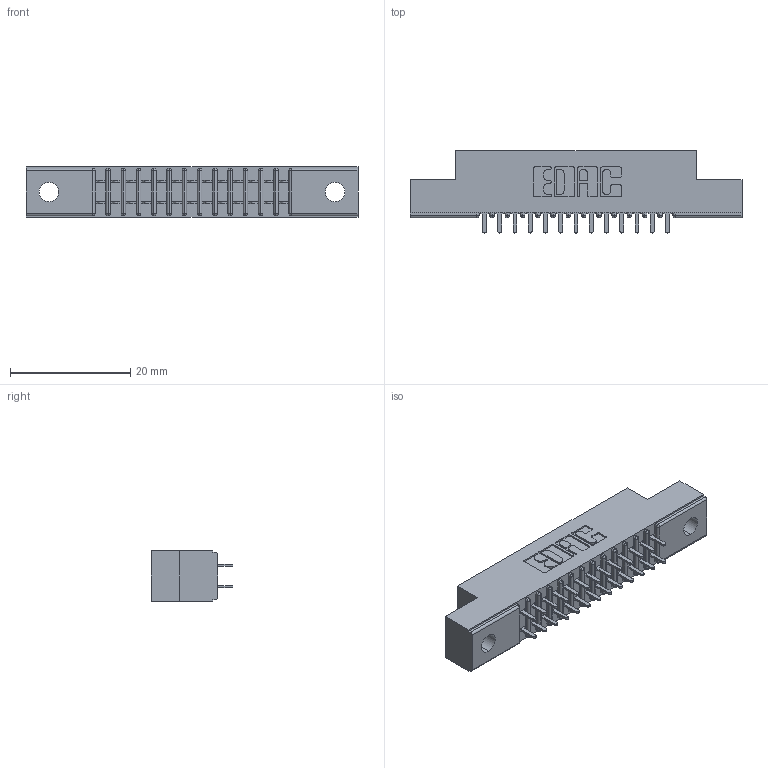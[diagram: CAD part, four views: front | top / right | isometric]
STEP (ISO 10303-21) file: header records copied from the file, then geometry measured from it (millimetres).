
FILE_DESCRIPTION (( 'STEP AP203' ), '1' );
FILE_NAME ('391-026-524-202.STEP', '2018-08-08T20:27:36', ( '' ), ( '' ), 'SwSTEP 2.0', 'SolidWorks 2016', '' );
FILE_SCHEMA (( 'CONFIG_CONTROL_DESIGN' ));
Length unit declared in the file: inch
Products named in the file (3): 341 Part_.128 (3.25) Dia Mounting Holes; 341-292-001_341-292-124; 391-026-524-202
Assembly tree (27 placements, depth 2):
  391-026-524-202
    341 Part_.128 (3.25) Dia Mounting Holes
    341-292-001_341-292-124  x26
Bounding box: 55.24 x 13.64 x 8.38 mm (x, y, z)
Volume: 3127.1 mm3; surface area: 5671.1 mm2
Topology: 27 solids, 27 shells, 1832 faces, 5295 edges, 3430 vertices
Faces by surface type: plane 1108, cylinder 672, sphere 28, torus 24
Entity records: 19598 total; most frequent: CARTESIAN_POINT 3259, ORIENTED_EDGE 3234, DIRECTION 3183, EDGE_CURVE 1617, LINE 1275, VECTOR 1275, VERTEX_POINT 1030, AXIS2_PLACEMENT_3D 954
